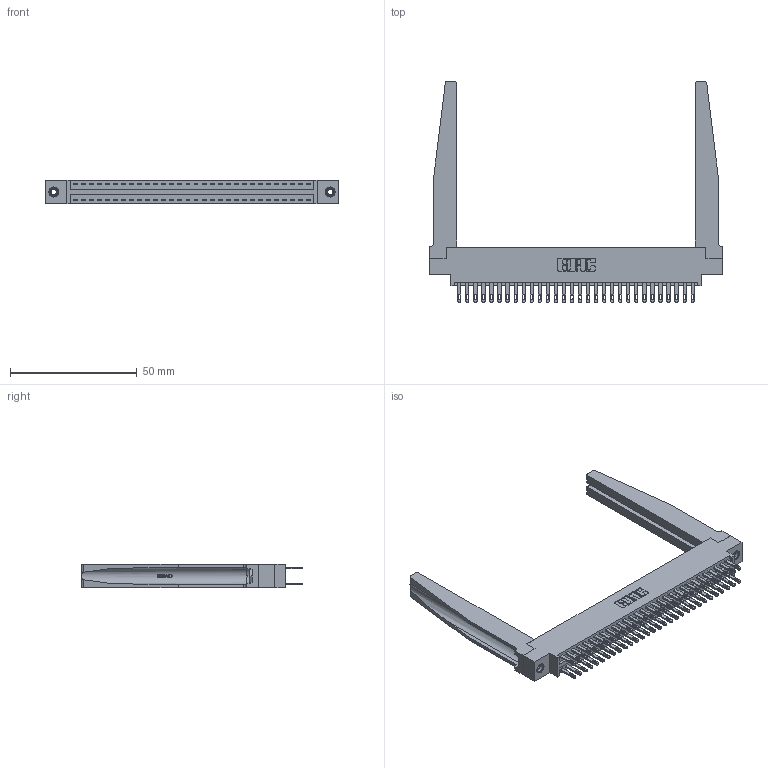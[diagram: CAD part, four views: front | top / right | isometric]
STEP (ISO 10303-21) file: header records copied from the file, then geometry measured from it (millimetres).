
FILE_DESCRIPTION (( 'STEP AP203' ), '1' );
FILE_NAME ('346-060-500-878.STEP', '2022-05-21T10:15:16', ( '' ), ( '' ), 'SwSTEP 2.0', 'SolidWorks 2020', '' );
FILE_SCHEMA (( 'CONFIG_CONTROL_DESIGN' ));
Length unit declared in the file: inch
Products named in the file (5): 346-220-078_345-220-078; 346 Part_0.170 Offset - 0.156 Dia-TH; 346-060-500-878; 345-250-001_345-250-001-102; 345-292-001_345-293-100
Assembly tree (65 placements, depth 2):
  346-060-500-878
    346 Part_0.170 Offset - 0.156 Dia-TH
    345-292-001_345-293-100  x60
    346-220-078_345-220-078  x2
    345-250-001_345-250-001-102  x2
Bounding box: 115.82 x 87.12 x 9.4 mm (x, y, z)
Volume: 18120.6 mm3; surface area: 22602.3 mm2
Topology: 65 solids, 65 shells, 3254 faces, 9805 edges, 6526 vertices
Faces by surface type: plane 1976, cylinder 1226, bspline 36, cone 12, torus 4
Entity records: 26420 total; most frequent: CARTESIAN_POINT 5313, ORIENTED_EDGE 4134, DIRECTION 3721, EDGE_CURVE 2067, VECTOR 1717, LINE 1717, VERTEX_POINT 1372, AXIS2_PLACEMENT_3D 1002
